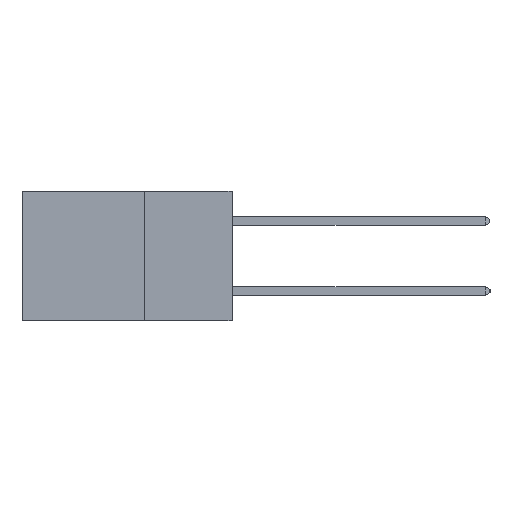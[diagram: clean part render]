
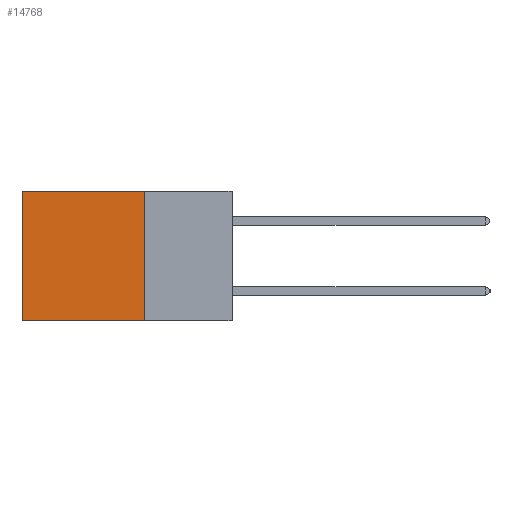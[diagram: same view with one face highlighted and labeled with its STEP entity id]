
A CAD part, left-side view. The second image highlights one B-rep face of the part: STEP entity #14768.
In plain terms, the highlighted planar face has unit normal (-1, 0, 0).
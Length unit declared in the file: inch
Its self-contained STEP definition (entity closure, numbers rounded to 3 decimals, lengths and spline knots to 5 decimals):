
#371 = FACE_OUTER_BOUND ( 'NONE', #10005, .T. ) ;
#548 = LINE ( 'NONE', #17270, #18068 ) ;
#598 = CARTESIAN_POINT ( 'NONE',  ( 0.2875, 0.6, -0.37 ) ) ;
#2420 = ORIENTED_EDGE ( 'NONE', *, *, #4250, .F. ) ;
#2910 = VECTOR ( 'NONE', #20865, 39.37008 ) ;
#3825 = DIRECTION ( 'NONE',  ( 0., 0., -1. ) ) ;
#4111 = ORIENTED_EDGE ( 'NONE', *, *, #15541, .F. ) ;
#4250 = EDGE_CURVE ( 'NONE', #8177, #5230, #19789, .T. ) ;
#4480 = DIRECTION ( 'NONE',  ( 0., 0., -1. ) ) ;
#5230 = VERTEX_POINT ( 'NONE', #598 ) ;
#6749 = CARTESIAN_POINT ( 'NONE',  ( 0.2875, 0.25, -0.37 ) ) ;
#7341 = EDGE_CURVE ( 'NONE', #13778, #13895, #7559, .T. ) ;
#7559 = LINE ( 'NONE', #7753, #2910 ) ;
#7578 = ORIENTED_EDGE ( 'NONE', *, *, #16683, .T. ) ;
#7705 = DIRECTION ( 'NONE',  ( 1., 0., 0. ) ) ;
#7753 = CARTESIAN_POINT ( 'NONE',  ( 0.2875, 0.25, 0. ) ) ;
#7973 = CARTESIAN_POINT ( 'NONE',  ( 0.2875, 0.25, 0. ) ) ;
#8177 = VERTEX_POINT ( 'NONE', #8487 ) ;
#8487 = CARTESIAN_POINT ( 'NONE',  ( 0.2875, 0.25, -0.37 ) ) ;
#10005 = EDGE_LOOP ( 'NONE', ( #7578, #2420, #4111, #10650 ) ) ;
#10650 = ORIENTED_EDGE ( 'NONE', *, *, #7341, .T. ) ;
#11207 = VECTOR ( 'NONE', #4480, 39.37008 ) ;
#11726 = LINE ( 'NONE', #7973, #11207 ) ;
#11761 = DIRECTION ( 'NONE',  ( 0., 1., 0. ) ) ;
#12652 = CARTESIAN_POINT ( 'NONE',  ( 0.2875, 0.25, 0. ) ) ;
#13778 = VERTEX_POINT ( 'NONE', #16597 ) ;
#13895 = VERTEX_POINT ( 'NONE', #19933 ) ;
#14768 = ADVANCED_FACE ( 'NONE', ( #371 ), #17609, .F. ) ;
#15541 = EDGE_CURVE ( 'NONE', #13778, #8177, #11726, .T. ) ;
#15621 = AXIS2_PLACEMENT_3D ( 'NONE', #12652, #7705, #19201 ) ;
#16551 = VECTOR ( 'NONE', #11761, 39.37008 ) ;
#16597 = CARTESIAN_POINT ( 'NONE',  ( 0.2875, 0.25, 0. ) ) ;
#16683 = EDGE_CURVE ( 'NONE', #13895, #5230, #548, .T. ) ;
#17270 = CARTESIAN_POINT ( 'NONE',  ( 0.2875, 0.6, 0. ) ) ;
#17609 = PLANE ( 'NONE',  #15621 ) ;
#18068 = VECTOR ( 'NONE', #3825, 39.37008 ) ;
#19201 = DIRECTION ( 'NONE',  ( 0., 0., -1. ) ) ;
#19789 = LINE ( 'NONE', #6749, #16551 ) ;
#19933 = CARTESIAN_POINT ( 'NONE',  ( 0.2875, 0.6, 0. ) ) ;
#20865 = DIRECTION ( 'NONE',  ( 0., 1., 0. ) ) ;
